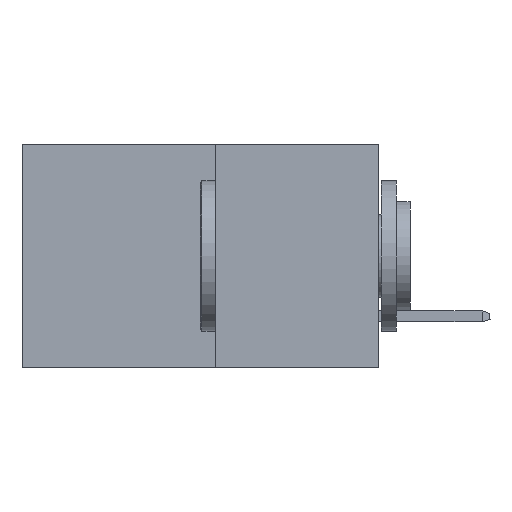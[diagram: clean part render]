
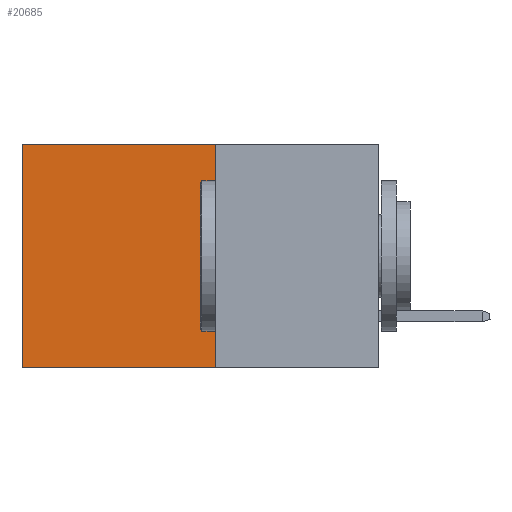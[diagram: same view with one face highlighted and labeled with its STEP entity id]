
A CAD part, left-side view. The second image highlights one B-rep face of the part: STEP entity #20685.
In plain terms, the highlighted planar face has unit normal (-1, 0, 0).
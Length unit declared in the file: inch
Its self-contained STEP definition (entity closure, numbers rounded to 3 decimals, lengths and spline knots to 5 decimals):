
#2827 = LINE ( 'NONE', #11007, #12181 ) ;
#3342 = VERTEX_POINT ( 'NONE', #13910 ) ;
#3567 = EDGE_CURVE ( 'NONE', #16495, #20190, #13694, .T. ) ;
#3797 = CARTESIAN_POINT ( 'NONE',  ( 0.277, 0.27, 0. ) ) ;
#4372 = ORIENTED_EDGE ( 'NONE', *, *, #6556, .F. ) ;
#4856 = DIRECTION ( 'NONE',  ( 0., 1., 0. ) ) ;
#5660 = FACE_OUTER_BOUND ( 'NONE', #11640, .T. ) ;
#6556 = EDGE_CURVE ( 'NONE', #16495, #3342, #13537, .T. ) ;
#6793 = PLANE ( 'NONE',  #19293 ) ;
#7004 = ORIENTED_EDGE ( 'NONE', *, *, #3567, .T. ) ;
#7292 = CARTESIAN_POINT ( 'NONE',  ( 0.277, 0.27, -0.37 ) ) ;
#7299 = ORIENTED_EDGE ( 'NONE', *, *, #19941, .T. ) ;
#8472 = VECTOR ( 'NONE', #11251, 39.37008 ) ;
#8685 = DIRECTION ( 'NONE',  ( 1., 0., 0. ) ) ;
#9579 = EDGE_CURVE ( 'NONE', #3342, #9883, #18689, .T. ) ;
#9883 = VERTEX_POINT ( 'NONE', #17481 ) ;
#11007 = CARTESIAN_POINT ( 'NONE',  ( 0.277, 0.59, -0.37 ) ) ;
#11096 = DIRECTION ( 'NONE',  ( 0., 1., 0. ) ) ;
#11251 = DIRECTION ( 'NONE',  ( 0., 0., -1. ) ) ;
#11302 = CARTESIAN_POINT ( 'NONE',  ( 0.277, 0.27, -0.37 ) ) ;
#11640 = EDGE_LOOP ( 'NONE', ( #7299, #16751, #4372, #7004 ) ) ;
#12181 = VECTOR ( 'NONE', #12931, 39.37008 ) ;
#12931 = DIRECTION ( 'NONE',  ( 0., 0., -1. ) ) ;
#13537 = LINE ( 'NONE', #11302, #8472 ) ;
#13694 = LINE ( 'NONE', #3797, #22811 ) ;
#13910 = CARTESIAN_POINT ( 'NONE',  ( 0.277, 0.27, -0.37 ) ) ;
#16495 = VERTEX_POINT ( 'NONE', #21271 ) ;
#16751 = ORIENTED_EDGE ( 'NONE', *, *, #9579, .F. ) ;
#17481 = CARTESIAN_POINT ( 'NONE',  ( 0.277, 0.59, -0.37 ) ) ;
#18689 = LINE ( 'NONE', #7292, #22891 ) ;
#19293 = AXIS2_PLACEMENT_3D ( 'NONE', #19849, #8685, #21657 ) ;
#19849 = CARTESIAN_POINT ( 'NONE',  ( 0.277, 0.27, -0.37 ) ) ;
#19941 = EDGE_CURVE ( 'NONE', #20190, #9883, #2827, .T. ) ;
#20190 = VERTEX_POINT ( 'NONE', #20954 ) ;
#20685 = ADVANCED_FACE ( 'NONE', ( #5660 ), #6793, .F. ) ;
#20954 = CARTESIAN_POINT ( 'NONE',  ( 0.277, 0.59, 0. ) ) ;
#21271 = CARTESIAN_POINT ( 'NONE',  ( 0.277, 0.27, 0. ) ) ;
#21657 = DIRECTION ( 'NONE',  ( 0., 0., -1. ) ) ;
#22811 = VECTOR ( 'NONE', #4856, 39.37008 ) ;
#22891 = VECTOR ( 'NONE', #11096, 39.37008 ) ;
